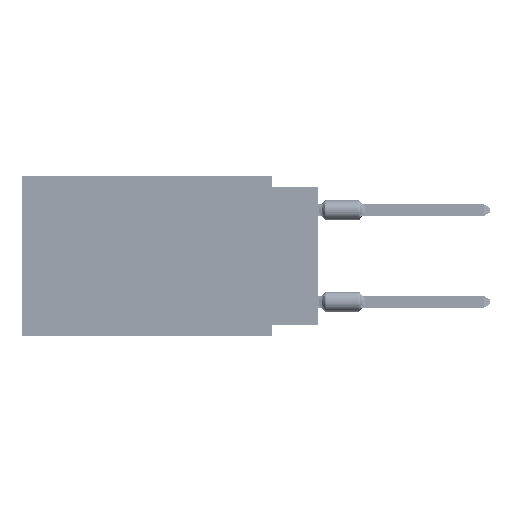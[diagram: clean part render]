
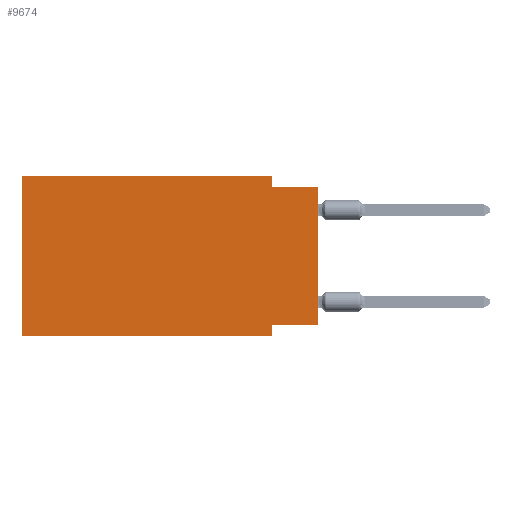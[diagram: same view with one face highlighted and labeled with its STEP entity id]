
A CAD part, left-side view. The second image highlights one B-rep face of the part: STEP entity #9674.
In plain terms, the highlighted planar face has unit normal (-1, 0, 0).
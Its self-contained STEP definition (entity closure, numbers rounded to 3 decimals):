
#93 = VECTOR ( 'NONE', #1965, 1000. ) ;
#511 = VECTOR ( 'NONE', #17472, 1000. ) ;
#952 = DIRECTION ( 'NONE',  ( 0., -1., 0. ) ) ;
#1149 = LINE ( 'NONE', #57294, #55296 ) ;
#1965 = DIRECTION ( 'NONE',  ( 0., 0., -1. ) ) ;
#2168 = CARTESIAN_POINT ( 'NONE',  ( 0., 2.54, -0.635 ) ) ;
#2320 = VERTEX_POINT ( 'NONE', #59091 ) ;
#3245 = VECTOR ( 'NONE', #8348, 1000. ) ;
#6455 = DIRECTION ( 'NONE',  ( 0., -1., 0. ) ) ;
#6707 = VERTEX_POINT ( 'NONE', #62377 ) ;
#6973 = LINE ( 'NONE', #47740, #93 ) ;
#7013 = VECTOR ( 'NONE', #32263, 1000. ) ;
#8188 = CARTESIAN_POINT ( 'NONE',  ( 0., 16.383, 0. ) ) ;
#8348 = DIRECTION ( 'NONE',  ( 0., 0., -1. ) ) ;
#8604 = PLANE ( 'NONE',  #35117 ) ;
#8674 = EDGE_CURVE ( 'NONE', #21632, #23599, #11863, .T. ) ;
#8969 = ORIENTED_EDGE ( 'NONE', *, *, #9049, .F. ) ;
#9049 = EDGE_CURVE ( 'NONE', #43152, #23599, #20840, .T. ) ;
#9243 = DIRECTION ( 'NONE',  ( 1., 0., 0. ) ) ;
#9674 = ADVANCED_FACE ( 'NONE', ( #48699 ), #8604, .F. ) ;
#9736 = VERTEX_POINT ( 'NONE', #24633 ) ;
#10274 = EDGE_CURVE ( 'NONE', #6707, #57450, #27175, .T. ) ;
#11103 = EDGE_CURVE ( 'NONE', #6707, #2320, #51756, .T. ) ;
#11273 = VERTEX_POINT ( 'NONE', #22990 ) ;
#11863 = LINE ( 'NONE', #63336, #7013 ) ;
#12406 = ORIENTED_EDGE ( 'NONE', *, *, #11103, .T. ) ;
#13351 = CARTESIAN_POINT ( 'NONE',  ( 0., 2.54, -8.89 ) ) ;
#15243 = CARTESIAN_POINT ( 'NONE',  ( 0., 0., -0.635 ) ) ;
#17472 = DIRECTION ( 'NONE',  ( 0., 0., 1. ) ) ;
#17972 = ORIENTED_EDGE ( 'NONE', *, *, #65135, .F. ) ;
#18958 = ORIENTED_EDGE ( 'NONE', *, *, #10274, .F. ) ;
#20694 = CARTESIAN_POINT ( 'NONE',  ( 0., 16.383, -8.89 ) ) ;
#20840 = LINE ( 'NONE', #32190, #39080 ) ;
#21632 = VERTEX_POINT ( 'NONE', #27742 ) ;
#22990 = CARTESIAN_POINT ( 'NONE',  ( 0., 2.54, 0. ) ) ;
#23599 = VERTEX_POINT ( 'NONE', #15243 ) ;
#23643 = DIRECTION ( 'NONE',  ( 0., 0., -1. ) ) ;
#23683 = ORIENTED_EDGE ( 'NONE', *, *, #8674, .T. ) ;
#24056 = ORIENTED_EDGE ( 'NONE', *, *, #24618, .F. ) ;
#24618 = EDGE_CURVE ( 'NONE', #11273, #43152, #6973, .T. ) ;
#24633 = CARTESIAN_POINT ( 'NONE',  ( 0., 2.54, -8.255 ) ) ;
#24946 = LINE ( 'NONE', #45326, #65122 ) ;
#27175 = LINE ( 'NONE', #41907, #511 ) ;
#27742 = CARTESIAN_POINT ( 'NONE',  ( 0., 0., -8.255 ) ) ;
#32190 = CARTESIAN_POINT ( 'NONE',  ( 0., 0., -0.635 ) ) ;
#32263 = DIRECTION ( 'NONE',  ( 0., 0., 1. ) ) ;
#35117 = AXIS2_PLACEMENT_3D ( 'NONE', #59719, #9243, #23643 ) ;
#35775 = EDGE_CURVE ( 'NONE', #9736, #2320, #58829, .T. ) ;
#39080 = VECTOR ( 'NONE', #6455, 1000. ) ;
#39957 = ORIENTED_EDGE ( 'NONE', *, *, #35775, .F. ) ;
#40810 = ORIENTED_EDGE ( 'NONE', *, *, #61246, .F. ) ;
#41907 = CARTESIAN_POINT ( 'NONE',  ( 0., 16.383, 0. ) ) ;
#41932 = DIRECTION ( 'NONE',  ( 0., 1., 0. ) ) ;
#43152 = VERTEX_POINT ( 'NONE', #2168 ) ;
#45326 = CARTESIAN_POINT ( 'NONE',  ( 0., 16.383, 0. ) ) ;
#47740 = CARTESIAN_POINT ( 'NONE',  ( 0., 2.54, 0. ) ) ;
#48699 = FACE_OUTER_BOUND ( 'NONE', #50208, .T. ) ;
#50208 = EDGE_LOOP ( 'NONE', ( #23683, #8969, #24056, #17972, #18958, #12406, #39957, #40810 ) ) ;
#51645 = VECTOR ( 'NONE', #952, 1000. ) ;
#51756 = LINE ( 'NONE', #20694, #51645 ) ;
#55296 = VECTOR ( 'NONE', #41932, 1000. ) ;
#57294 = CARTESIAN_POINT ( 'NONE',  ( 0., 0., -8.255 ) ) ;
#57450 = VERTEX_POINT ( 'NONE', #8188 ) ;
#58829 = LINE ( 'NONE', #13351, #3245 ) ;
#59091 = CARTESIAN_POINT ( 'NONE',  ( 0., 2.54, -8.89 ) ) ;
#59719 = CARTESIAN_POINT ( 'NONE',  ( 0., 16.383, 0. ) ) ;
#61246 = EDGE_CURVE ( 'NONE', #21632, #9736, #1149, .T. ) ;
#62377 = CARTESIAN_POINT ( 'NONE',  ( 0., 16.383, -8.89 ) ) ;
#63336 = CARTESIAN_POINT ( 'NONE',  ( 0., 0., 0. ) ) ;
#65122 = VECTOR ( 'NONE', #65721, 1000. ) ;
#65135 = EDGE_CURVE ( 'NONE', #57450, #11273, #24946, .T. ) ;
#65721 = DIRECTION ( 'NONE',  ( 0., -1., 0. ) ) ;
